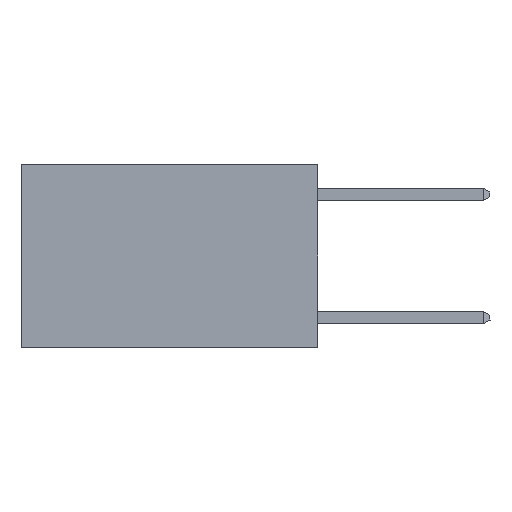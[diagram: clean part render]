
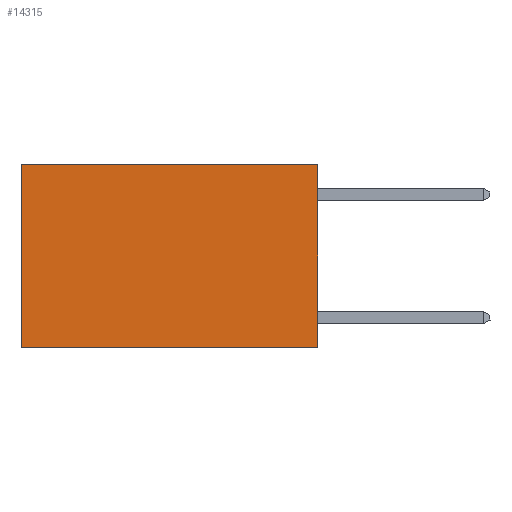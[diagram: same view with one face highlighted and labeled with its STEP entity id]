
A CAD part, left-side view. The second image highlights one B-rep face of the part: STEP entity #14315.
In plain terms, the highlighted planar face has unit normal (-1, 0, 0).
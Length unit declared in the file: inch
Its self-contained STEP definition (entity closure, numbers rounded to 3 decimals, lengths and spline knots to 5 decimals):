
#81 = ORIENTED_EDGE ( 'NONE', *, *, #23672, .T. ) ;
#298 = ORIENTED_EDGE ( 'NONE', *, *, #25483, .F. ) ;
#723 = DIRECTION ( 'NONE',  ( 0., 0., -1. ) ) ;
#1425 = VECTOR ( 'NONE', #18855, 39.37008 ) ;
#1793 = EDGE_LOOP ( 'NONE', ( #81, #298, #14492, #8347 ) ) ;
#1814 = CARTESIAN_POINT ( 'NONE',  ( 0.2625, 0., -0.37 ) ) ;
#1853 = VECTOR ( 'NONE', #21205, 39.37008 ) ;
#2107 = LINE ( 'NONE', #4089, #1425 ) ;
#4089 = CARTESIAN_POINT ( 'NONE',  ( 0.2625, 0.6, 0. ) ) ;
#4428 = CARTESIAN_POINT ( 'NONE',  ( 0.2625, 0., 0. ) ) ;
#4877 = CARTESIAN_POINT ( 'NONE',  ( 0.2625, 0., 0. ) ) ;
#5170 = FACE_OUTER_BOUND ( 'NONE', #1793, .T. ) ;
#6065 = VERTEX_POINT ( 'NONE', #11744 ) ;
#6835 = CARTESIAN_POINT ( 'NONE',  ( 0.2625, 0., 0. ) ) ;
#6853 = AXIS2_PLACEMENT_3D ( 'NONE', #4877, #13320, #723 ) ;
#6919 = LINE ( 'NONE', #10745, #11847 ) ;
#8347 = ORIENTED_EDGE ( 'NONE', *, *, #9700, .T. ) ;
#9700 = EDGE_CURVE ( 'NONE', #14784, #16175, #25187, .T. ) ;
#10745 = CARTESIAN_POINT ( 'NONE',  ( 0.2625, 0., -0.37 ) ) ;
#11744 = CARTESIAN_POINT ( 'NONE',  ( 0.2625, 0.6, -0.37 ) ) ;
#11847 = VECTOR ( 'NONE', #17116, 39.37008 ) ;
#13008 = LINE ( 'NONE', #4428, #1853 ) ;
#13320 = DIRECTION ( 'NONE',  ( 1., 0., 0. ) ) ;
#14315 = ADVANCED_FACE ( 'NONE', ( #5170 ), #25878, .F. ) ;
#14492 = ORIENTED_EDGE ( 'NONE', *, *, #14905, .F. ) ;
#14647 = VECTOR ( 'NONE', #19431, 39.37008 ) ;
#14784 = VERTEX_POINT ( 'NONE', #16621 ) ;
#14905 = EDGE_CURVE ( 'NONE', #14784, #22860, #13008, .T. ) ;
#16175 = VERTEX_POINT ( 'NONE', #18858 ) ;
#16621 = CARTESIAN_POINT ( 'NONE',  ( 0.2625, 0., 0. ) ) ;
#17116 = DIRECTION ( 'NONE',  ( 0., 1., 0. ) ) ;
#18855 = DIRECTION ( 'NONE',  ( 0., 0., -1. ) ) ;
#18858 = CARTESIAN_POINT ( 'NONE',  ( 0.2625, 0.6, 0. ) ) ;
#19431 = DIRECTION ( 'NONE',  ( 0., 1., 0. ) ) ;
#21205 = DIRECTION ( 'NONE',  ( 0., 0., -1. ) ) ;
#22860 = VERTEX_POINT ( 'NONE', #1814 ) ;
#23672 = EDGE_CURVE ( 'NONE', #16175, #6065, #2107, .T. ) ;
#25187 = LINE ( 'NONE', #6835, #14647 ) ;
#25483 = EDGE_CURVE ( 'NONE', #22860, #6065, #6919, .T. ) ;
#25878 = PLANE ( 'NONE',  #6853 ) ;
